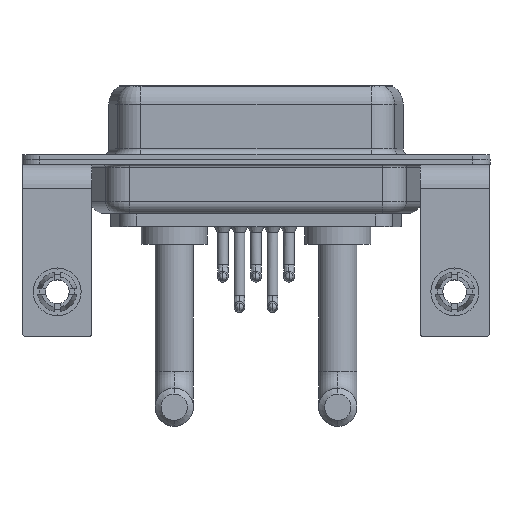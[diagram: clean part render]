
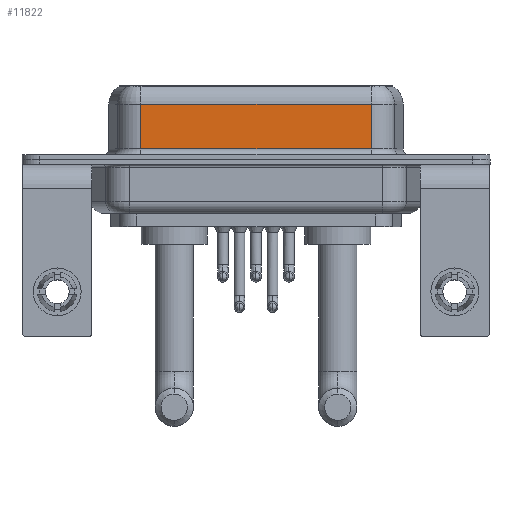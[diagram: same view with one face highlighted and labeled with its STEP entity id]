
A CAD part, front view. The second image highlights one B-rep face of the part: STEP entity #11822.
In plain terms, the highlighted planar face has unit normal (0, -1, 0).
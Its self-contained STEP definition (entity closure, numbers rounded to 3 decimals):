
#486 = VERTEX_POINT ( 'NONE', #2633 ) ;
#1450 = DIRECTION ( 'NONE',  ( 0., 1., 0. ) ) ;
#1480 = CARTESIAN_POINT ( 'NONE',  ( 26.287, -3.95, 0.9 ) ) ;
#1581 = AXIS2_PLACEMENT_3D ( 'NONE', #18830, #1450, #5491 ) ;
#2323 = ORIENTED_EDGE ( 'NONE', *, *, #5924, .T. ) ;
#2633 = CARTESIAN_POINT ( 'NONE',  ( 26.287, -3.95, 4.65 ) ) ;
#3358 = CARTESIAN_POINT ( 'NONE',  ( 26.287, -3.95, 0.9 ) ) ;
#3794 = CARTESIAN_POINT ( 'NONE',  ( 26.287, -3.95, 6.4 ) ) ;
#4794 = EDGE_CURVE ( 'NONE', #486, #8542, #9402, .T. ) ;
#5086 = DIRECTION ( 'NONE',  ( 0., 0., -1. ) ) ;
#5307 = EDGE_CURVE ( 'NONE', #486, #18305, #15429, .T. ) ;
#5491 = DIRECTION ( 'NONE',  ( 0., 0., 1. ) ) ;
#5924 = EDGE_CURVE ( 'NONE', #12821, #18305, #10493, .T. ) ;
#6410 = VECTOR ( 'NONE', #18326, 1000. ) ;
#6953 = FACE_OUTER_BOUND ( 'NONE', #12096, .T. ) ;
#7307 = ORIENTED_EDGE ( 'NONE', *, *, #4794, .T. ) ;
#7839 = CARTESIAN_POINT ( 'NONE',  ( 26.287, -3.95, 4.65 ) ) ;
#8542 = VERTEX_POINT ( 'NONE', #19107 ) ;
#9402 = LINE ( 'NONE', #7839, #15704 ) ;
#10174 = VECTOR ( 'NONE', #12054, 1000. ) ;
#10493 = LINE ( 'NONE', #3358, #10174 ) ;
#10534 = PLANE ( 'NONE',  #1581 ) ;
#10575 = DIRECTION ( 'NONE',  ( -1., 0., 0. ) ) ;
#11822 = ADVANCED_FACE ( 'NONE', ( #6953 ), #10534, .F. ) ;
#12054 = DIRECTION ( 'NONE',  ( 1., 0., 0. ) ) ;
#12096 = EDGE_LOOP ( 'NONE', ( #15091, #7307, #18802, #2323 ) ) ;
#12788 = LINE ( 'NONE', #13868, #14374 ) ;
#12821 = VERTEX_POINT ( 'NONE', #17980 ) ;
#13414 = EDGE_CURVE ( 'NONE', #8542, #12821, #12788, .T. ) ;
#13868 = CARTESIAN_POINT ( 'NONE',  ( 7.013, -3.95, 6.4 ) ) ;
#14374 = VECTOR ( 'NONE', #5086, 1000. ) ;
#15091 = ORIENTED_EDGE ( 'NONE', *, *, #5307, .F. ) ;
#15429 = LINE ( 'NONE', #3794, #6410 ) ;
#15704 = VECTOR ( 'NONE', #10575, 1000. ) ;
#17980 = CARTESIAN_POINT ( 'NONE',  ( 7.013, -3.95, 0.9 ) ) ;
#18305 = VERTEX_POINT ( 'NONE', #1480 ) ;
#18326 = DIRECTION ( 'NONE',  ( 0., 0., -1. ) ) ;
#18802 = ORIENTED_EDGE ( 'NONE', *, *, #13414, .T. ) ;
#18830 = CARTESIAN_POINT ( 'NONE',  ( 26.287, -3.95, 6.4 ) ) ;
#19107 = CARTESIAN_POINT ( 'NONE',  ( 7.013, -3.95, 4.65 ) ) ;
